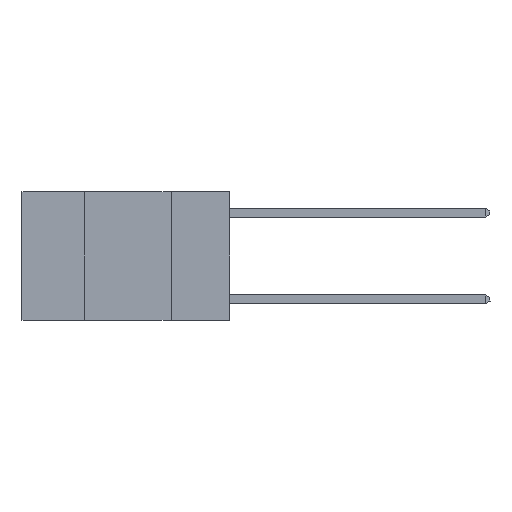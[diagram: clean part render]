
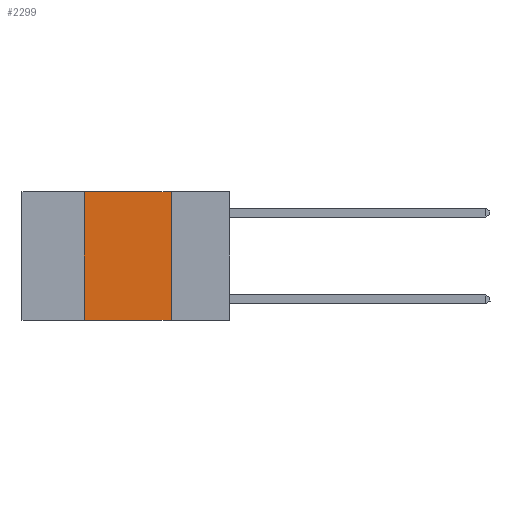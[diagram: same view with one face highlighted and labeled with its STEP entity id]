
A CAD part, left-side view. The second image highlights one B-rep face of the part: STEP entity #2299.
In plain terms, the highlighted planar face has unit normal (-1, 0, 0).
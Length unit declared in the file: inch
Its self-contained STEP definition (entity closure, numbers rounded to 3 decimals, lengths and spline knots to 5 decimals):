
#146 = ORIENTED_EDGE ( 'NONE', *, *, #553, .F. ) ;
#367 = ORIENTED_EDGE ( 'NONE', *, *, #4144, .F. ) ;
#468 = PLANE ( 'NONE',  #4846 ) ;
#553 = EDGE_CURVE ( 'NONE', #7750, #6968, #2398, .T. ) ;
#822 = LINE ( 'NONE', #7575, #7950 ) ;
#1193 = CARTESIAN_POINT ( 'NONE',  ( 0., 0.17, 0. ) ) ;
#1265 = VERTEX_POINT ( 'NONE', #2716 ) ;
#1812 = LINE ( 'NONE', #7899, #8684 ) ;
#2229 = ORIENTED_EDGE ( 'NONE', *, *, #7098, .T. ) ;
#2299 = ADVANCED_FACE ( 'NONE', ( #2718 ), #468, .F. ) ;
#2398 = LINE ( 'NONE', #3391, #3839 ) ;
#2429 = DIRECTION ( 'NONE',  ( 0., 0., -1. ) ) ;
#2716 = CARTESIAN_POINT ( 'NONE',  ( 0., 0.42, -0.37 ) ) ;
#2718 = FACE_OUTER_BOUND ( 'NONE', #2858, .T. ) ;
#2757 = DIRECTION ( 'NONE',  ( 1., 0., 0. ) ) ;
#2858 = EDGE_LOOP ( 'NONE', ( #367, #146, #4102, #2229 ) ) ;
#2943 = VECTOR ( 'NONE', #5361, 39.37008 ) ;
#3391 = CARTESIAN_POINT ( 'NONE',  ( 0., 0.6, 0. ) ) ;
#3839 = VECTOR ( 'NONE', #4524, 39.37008 ) ;
#3933 = CARTESIAN_POINT ( 'NONE',  ( 0., 0.6, 0. ) ) ;
#4102 = ORIENTED_EDGE ( 'NONE', *, *, #6333, .F. ) ;
#4144 = EDGE_CURVE ( 'NONE', #6968, #8448, #4805, .T. ) ;
#4524 = DIRECTION ( 'NONE',  ( 0., -1., 0. ) ) ;
#4805 = LINE ( 'NONE', #6032, #2943 ) ;
#4846 = AXIS2_PLACEMENT_3D ( 'NONE', #3933, #2757, #2429 ) ;
#5361 = DIRECTION ( 'NONE',  ( 0., 0., -1. ) ) ;
#6032 = CARTESIAN_POINT ( 'NONE',  ( 0., 0.17, 0. ) ) ;
#6206 = CARTESIAN_POINT ( 'NONE',  ( 0., 0.17, -0.37 ) ) ;
#6333 = EDGE_CURVE ( 'NONE', #1265, #7750, #1812, .T. ) ;
#6968 = VERTEX_POINT ( 'NONE', #1193 ) ;
#7098 = EDGE_CURVE ( 'NONE', #1265, #8448, #822, .T. ) ;
#7575 = CARTESIAN_POINT ( 'NONE',  ( 0., 0.6, -0.37 ) ) ;
#7750 = VERTEX_POINT ( 'NONE', #8207 ) ;
#7899 = CARTESIAN_POINT ( 'NONE',  ( 0., 0.42, 0. ) ) ;
#7950 = VECTOR ( 'NONE', #8245, 39.37008 ) ;
#8207 = CARTESIAN_POINT ( 'NONE',  ( 0., 0.42, 0. ) ) ;
#8245 = DIRECTION ( 'NONE',  ( 0., -1., 0. ) ) ;
#8448 = VERTEX_POINT ( 'NONE', #6206 ) ;
#8563 = DIRECTION ( 'NONE',  ( 0., 0., 1. ) ) ;
#8684 = VECTOR ( 'NONE', #8563, 39.37008 ) ;
